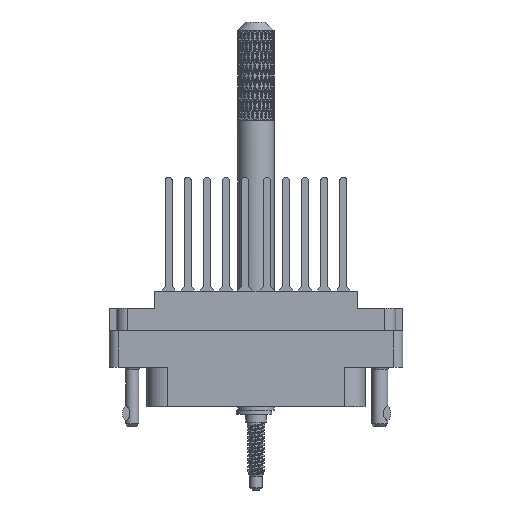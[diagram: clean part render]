
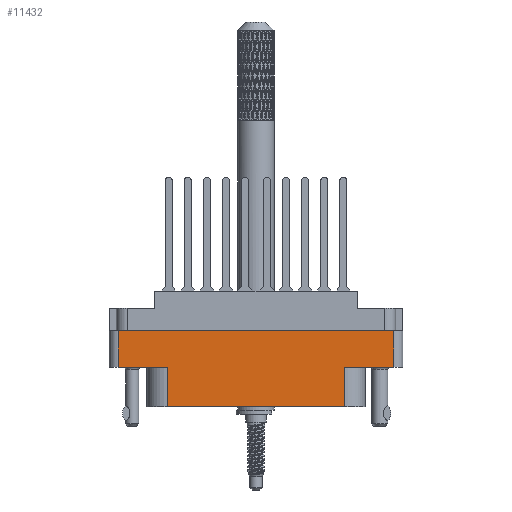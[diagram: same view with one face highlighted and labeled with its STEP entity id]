
A CAD part, front view. The second image highlights one B-rep face of the part: STEP entity #11432.
In plain terms, the highlighted planar face has unit normal (0, -1, 0).
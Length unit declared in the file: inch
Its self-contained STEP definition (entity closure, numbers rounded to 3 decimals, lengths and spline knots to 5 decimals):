
#1062 = EDGE_CURVE ( 'NONE', #53724, #94225, #49970, .T. ) ;
#2109 = VERTEX_POINT ( 'NONE', #67829 ) ;
#2818 = EDGE_CURVE ( 'NONE', #87589, #2109, #106995, .T. ) ;
#6035 = VERTEX_POINT ( 'NONE', #14308 ) ;
#11432 = ADVANCED_FACE ( 'NONE', ( #111311 ), #108993, .T. ) ;
#11564 = LINE ( 'NONE', #106565, #67294 ) ;
#12412 = CARTESIAN_POINT ( 'NONE',  ( -1., -0.438, -0.789 ) ) ;
#14308 = CARTESIAN_POINT ( 'NONE',  ( -0.938, -0.438, -0.268 ) ) ;
#22110 = DIRECTION ( 'NONE',  ( -1., 0., 0. ) ) ;
#23727 = CARTESIAN_POINT ( 'NONE',  ( 0.938, -0.438, -0.789 ) ) ;
#24748 = VECTOR ( 'NONE', #54022, 39.37008 ) ;
#25278 = EDGE_CURVE ( 'NONE', #82159, #2109, #88041, .T. ) ;
#26517 = VECTOR ( 'NONE', #97452, 39.37008 ) ;
#28906 = CARTESIAN_POINT ( 'NONE',  ( -0.604, -0.438, -0.52 ) ) ;
#30675 = DIRECTION ( 'NONE',  ( 0., 0., -1. ) ) ;
#32318 = ORIENTED_EDGE ( 'NONE', *, *, #35762, .T. ) ;
#32352 = VECTOR ( 'NONE', #111910, 39.37008 ) ;
#35762 = EDGE_CURVE ( 'NONE', #6035, #53724, #11564, .T. ) ;
#37799 = EDGE_CURVE ( 'NONE', #94225, #106116, #90049, .T. ) ;
#38591 = ORIENTED_EDGE ( 'NONE', *, *, #1062, .T. ) ;
#41532 = LINE ( 'NONE', #51332, #45599 ) ;
#41798 = EDGE_LOOP ( 'NONE', ( #75997, #32318, #38591, #49990, #59135, #97186, #105815, #60748 ) ) ;
#44171 = DIRECTION ( 'NONE',  ( 0., 0., -1. ) ) ;
#44182 = LINE ( 'NONE', #97836, #26517 ) ;
#45599 = VECTOR ( 'NONE', #70001, 39.37008 ) ;
#48745 = EDGE_CURVE ( 'NONE', #6035, #65304, #44182, .T. ) ;
#49970 = LINE ( 'NONE', #51061, #32352 ) ;
#49990 = ORIENTED_EDGE ( 'NONE', *, *, #37799, .T. ) ;
#51061 = CARTESIAN_POINT ( 'NONE',  ( 0., -0.438, -0.52 ) ) ;
#51332 = CARTESIAN_POINT ( 'NONE',  ( -1., -0.438, -0.789 ) ) ;
#53724 = VERTEX_POINT ( 'NONE', #97553 ) ;
#54022 = DIRECTION ( 'NONE',  ( 0., 0., -1. ) ) ;
#55047 = AXIS2_PLACEMENT_3D ( 'NONE', #12412, #82803, #30675 ) ;
#59135 = ORIENTED_EDGE ( 'NONE', *, *, #84035, .T. ) ;
#60748 = ORIENTED_EDGE ( 'NONE', *, *, #103337, .T. ) ;
#64840 = VECTOR ( 'NONE', #22110, 39.37008 ) ;
#65304 = VERTEX_POINT ( 'NONE', #112575 ) ;
#67294 = VECTOR ( 'NONE', #44171, 39.37008 ) ;
#67829 = CARTESIAN_POINT ( 'NONE',  ( 0.604, -0.438, -0.52 ) ) ;
#70001 = DIRECTION ( 'NONE',  ( 1., 0., 0. ) ) ;
#75997 = ORIENTED_EDGE ( 'NONE', *, *, #48745, .F. ) ;
#76441 = VECTOR ( 'NONE', #85393, 39.37008 ) ;
#78486 = CARTESIAN_POINT ( 'NONE',  ( 0.604, -0.438, -0.52 ) ) ;
#82159 = VERTEX_POINT ( 'NONE', #86983 ) ;
#82803 = DIRECTION ( 'NONE',  ( 0., -1., 0. ) ) ;
#84035 = EDGE_CURVE ( 'NONE', #106116, #87589, #41532, .T. ) ;
#85393 = DIRECTION ( 'NONE',  ( 0., 0., 1. ) ) ;
#86983 = CARTESIAN_POINT ( 'NONE',  ( 0.938, -0.438, -0.52 ) ) ;
#87433 = LINE ( 'NONE', #23727, #76441 ) ;
#87589 = VERTEX_POINT ( 'NONE', #91154 ) ;
#88041 = LINE ( 'NONE', #107757, #64840 ) ;
#89343 = VECTOR ( 'NONE', #94530, 39.37008 ) ;
#90049 = LINE ( 'NONE', #95912, #24748 ) ;
#90963 = CARTESIAN_POINT ( 'NONE',  ( -0.604, -0.438, -0.789 ) ) ;
#91154 = CARTESIAN_POINT ( 'NONE',  ( 0.604, -0.438, -0.789 ) ) ;
#94225 = VERTEX_POINT ( 'NONE', #28906 ) ;
#94530 = DIRECTION ( 'NONE',  ( 0., 0., 1. ) ) ;
#95912 = CARTESIAN_POINT ( 'NONE',  ( -0.604, -0.438, -0.789 ) ) ;
#97186 = ORIENTED_EDGE ( 'NONE', *, *, #2818, .T. ) ;
#97452 = DIRECTION ( 'NONE',  ( 1., 0., 0. ) ) ;
#97553 = CARTESIAN_POINT ( 'NONE',  ( -0.938, -0.438, -0.52 ) ) ;
#97836 = CARTESIAN_POINT ( 'NONE',  ( 0., -0.438, -0.268 ) ) ;
#103337 = EDGE_CURVE ( 'NONE', #82159, #65304, #87433, .T. ) ;
#105815 = ORIENTED_EDGE ( 'NONE', *, *, #25278, .F. ) ;
#106116 = VERTEX_POINT ( 'NONE', #90963 ) ;
#106565 = CARTESIAN_POINT ( 'NONE',  ( -0.938, -0.438, -0.789 ) ) ;
#106995 = LINE ( 'NONE', #78486, #89343 ) ;
#107757 = CARTESIAN_POINT ( 'NONE',  ( 0., -0.438, -0.52 ) ) ;
#108993 = PLANE ( 'NONE',  #55047 ) ;
#111311 = FACE_OUTER_BOUND ( 'NONE', #41798, .T. ) ;
#111910 = DIRECTION ( 'NONE',  ( 1., 0., 0. ) ) ;
#112575 = CARTESIAN_POINT ( 'NONE',  ( 0.938, -0.438, -0.268 ) ) ;
